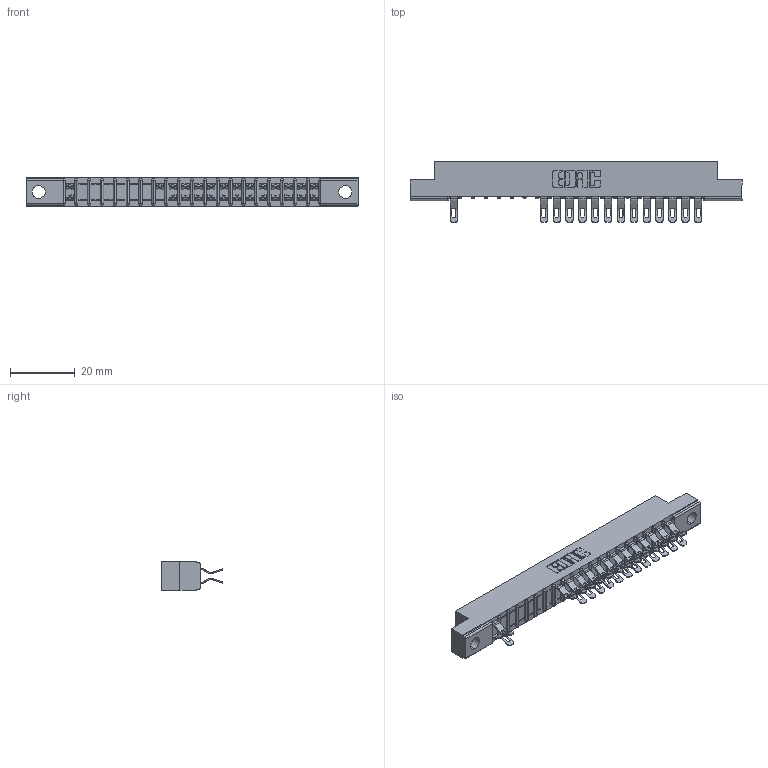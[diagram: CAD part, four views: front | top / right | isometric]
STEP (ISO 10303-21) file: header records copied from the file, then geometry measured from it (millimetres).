
FILE_DESCRIPTION (( 'STEP AP203' ), '1' );
FILE_NAME ('307-040-555-204.STEP', '2018-08-05T15:01:34', ( '' ), ( '' ), 'SwSTEP 2.0', 'SolidWorks 2016', '' );
FILE_SCHEMA (( 'CONFIG_CONTROL_DESIGN' ));
Length unit declared in the file: inch
Products named in the file (3): 307 Part_.156 Dia Mounting Holes; 307-290-001_555; 307-040-555-204
Assembly tree (28 placements, depth 2):
  307-040-555-204
    307 Part_.156 Dia Mounting Holes
    307-290-001_555  x27
Bounding box: 102.26 x 18.75 x 8.71 mm (x, y, z)
Volume: 6495.3 mm3; surface area: 10706.8 mm2
Topology: 28 solids, 28 shells, 1930 faces, 5662 edges, 3680 vertices
Faces by surface type: plane 1080, cylinder 808, sphere 42
Entity records: 21037 total; most frequent: CARTESIAN_POINT 3513, ORIENTED_EDGE 3492, DIRECTION 3436, EDGE_CURVE 1746, VECTOR 1326, LINE 1326, VERTEX_POINT 1132, AXIS2_PLACEMENT_3D 1055
